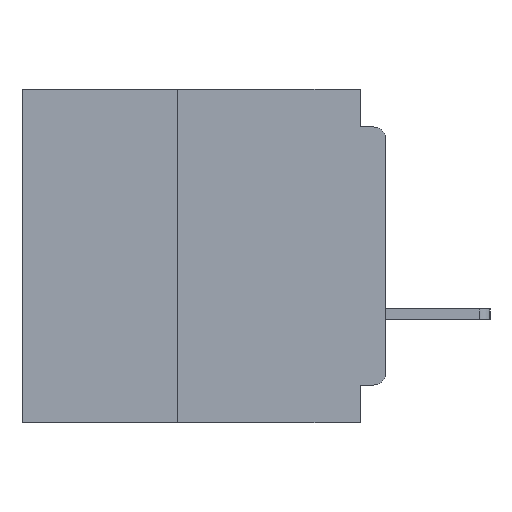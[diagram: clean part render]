
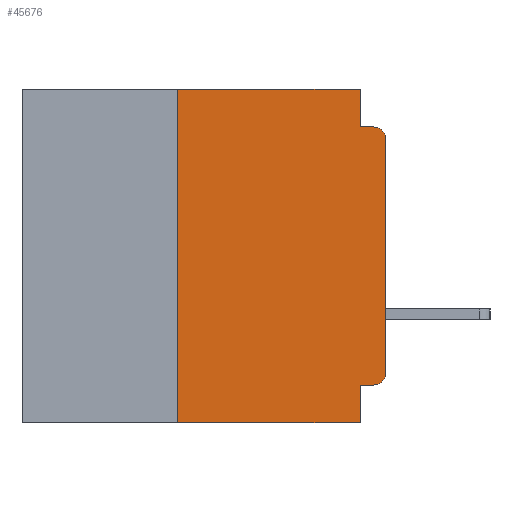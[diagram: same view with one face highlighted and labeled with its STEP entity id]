
A CAD part, left-side view. The second image highlights one B-rep face of the part: STEP entity #45676.
In plain terms, the highlighted planar face has unit normal (-1, 0, 0).
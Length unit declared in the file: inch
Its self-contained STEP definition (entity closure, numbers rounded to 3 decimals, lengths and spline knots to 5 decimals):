
#1343 = VECTOR ( 'NONE', #16385, 39.37008 ) ;
#1486 = CARTESIAN_POINT ( 'NONE',  ( 0., 0., -0.34 ) ) ;
#1702 = CARTESIAN_POINT ( 'NONE',  ( 0., 0.437, -0.4 ) ) ;
#2085 = CARTESIAN_POINT ( 'NONE',  ( 0., 0., -0.06 ) ) ;
#2551 = ORIENTED_EDGE ( 'NONE', *, *, #31045, .T. ) ;
#2575 = VERTEX_POINT ( 'NONE', #42273 ) ;
#2847 = CIRCLE ( 'NONE', #25628, 0.015 ) ;
#3550 = VERTEX_POINT ( 'NONE', #44899 ) ;
#4883 = ORIENTED_EDGE ( 'NONE', *, *, #26939, .T. ) ;
#7940 = CARTESIAN_POINT ( 'NONE',  ( 0., 0.25, -0.4 ) ) ;
#8504 = CARTESIAN_POINT ( 'NONE',  ( 0., 0.437, 0. ) ) ;
#9135 = CARTESIAN_POINT ( 'NONE',  ( 0., 0., -0.045 ) ) ;
#9590 = FACE_OUTER_BOUND ( 'NONE', #31355, .T. ) ;
#10597 = CARTESIAN_POINT ( 'NONE',  ( 0., 0.015, -0.34 ) ) ;
#11139 = CARTESIAN_POINT ( 'NONE',  ( 0., 0.015, -0.355 ) ) ;
#11684 = DIRECTION ( 'NONE',  ( 0., 0., -1. ) ) ;
#11767 = DIRECTION ( 'NONE',  ( 0., 0., 1. ) ) ;
#12786 = VERTEX_POINT ( 'NONE', #33466 ) ;
#12828 = DIRECTION ( 'NONE',  ( 0., -1., 0. ) ) ;
#13458 = DIRECTION ( 'NONE',  ( 0., -1., 0. ) ) ;
#14938 = DIRECTION ( 'NONE',  ( 0., 0., -1. ) ) ;
#15249 = EDGE_CURVE ( 'NONE', #35882, #40280, #45201, .T. ) ;
#16385 = DIRECTION ( 'NONE',  ( 0., 0., 1. ) ) ;
#16493 = AXIS2_PLACEMENT_3D ( 'NONE', #20084, #37190, #11684 ) ;
#18243 = VECTOR ( 'NONE', #52682, 39.37008 ) ;
#19333 = CARTESIAN_POINT ( 'NONE',  ( 0., 0.015, -0.06 ) ) ;
#20084 = CARTESIAN_POINT ( 'NONE',  ( 0., 0.437, 0. ) ) ;
#20311 = VERTEX_POINT ( 'NONE', #2085 ) ;
#21010 = DIRECTION ( 'NONE',  ( 0., 1., 0. ) ) ;
#22916 = DIRECTION ( 'NONE',  ( 0., -1., 0. ) ) ;
#23565 = DIRECTION ( 'NONE',  ( 0., 0., -1. ) ) ;
#23844 = VERTEX_POINT ( 'NONE', #30542 ) ;
#25628 = AXIS2_PLACEMENT_3D ( 'NONE', #10597, #40368, #14938 ) ;
#26117 = VECTOR ( 'NONE', #13458, 39.37008 ) ;
#26939 = EDGE_CURVE ( 'NONE', #43745, #46457, #2847, .T. ) ;
#28578 = ORIENTED_EDGE ( 'NONE', *, *, #34193, .T. ) ;
#30542 = CARTESIAN_POINT ( 'NONE',  ( 0., 0.031, 0. ) ) ;
#31045 = EDGE_CURVE ( 'NONE', #46457, #20311, #47578, .T. ) ;
#31355 = EDGE_LOOP ( 'NONE', ( #2551, #28578, #42741, #45619, #48476, #47615, #47704, #32924, #36792, #4883 ) ) ;
#31519 = CARTESIAN_POINT ( 'NONE',  ( 0., 0.031, -0.045 ) ) ;
#32924 = ORIENTED_EDGE ( 'NONE', *, *, #46124, .F. ) ;
#33305 = EDGE_CURVE ( 'NONE', #37287, #3550, #40085, .T. ) ;
#33466 = CARTESIAN_POINT ( 'NONE',  ( 0., 0.031, -0.355 ) ) ;
#33899 = LINE ( 'NONE', #42177, #35237 ) ;
#34193 = EDGE_CURVE ( 'NONE', #20311, #3550, #47916, .T. ) ;
#35237 = VECTOR ( 'NONE', #21010, 39.37008 ) ;
#35882 = VERTEX_POINT ( 'NONE', #51543 ) ;
#36351 = CARTESIAN_POINT ( 'NONE',  ( 0., 0.031, 0. ) ) ;
#36402 = VECTOR ( 'NONE', #11767, 39.37008 ) ;
#36792 = ORIENTED_EDGE ( 'NONE', *, *, #41934, .F. ) ;
#36910 = VECTOR ( 'NONE', #53026, 39.37008 ) ;
#37190 = DIRECTION ( 'NONE',  ( 1., 0., 0. ) ) ;
#37287 = VERTEX_POINT ( 'NONE', #31519 ) ;
#39342 = EDGE_CURVE ( 'NONE', #23844, #37287, #49363, .T. ) ;
#40085 = LINE ( 'NONE', #9135, #26117 ) ;
#40280 = VERTEX_POINT ( 'NONE', #42901 ) ;
#40368 = DIRECTION ( 'NONE',  ( -1., 0., 0. ) ) ;
#41226 = VECTOR ( 'NONE', #12828, 39.37008 ) ;
#41525 = CARTESIAN_POINT ( 'NONE',  ( 0., 0., 0. ) ) ;
#41934 = EDGE_CURVE ( 'NONE', #43745, #12786, #33899, .T. ) ;
#41965 = EDGE_CURVE ( 'NONE', #40280, #23844, #42528, .T. ) ;
#42177 = CARTESIAN_POINT ( 'NONE',  ( 0., 0., -0.355 ) ) ;
#42273 = CARTESIAN_POINT ( 'NONE',  ( 0., 0.031, -0.4 ) ) ;
#42528 = LINE ( 'NONE', #8504, #41226 ) ;
#42741 = ORIENTED_EDGE ( 'NONE', *, *, #33305, .F. ) ;
#42901 = CARTESIAN_POINT ( 'NONE',  ( 0., 0.25, 0. ) ) ;
#43745 = VERTEX_POINT ( 'NONE', #11139 ) ;
#44899 = CARTESIAN_POINT ( 'NONE',  ( 0., 0.015, -0.045 ) ) ;
#45201 = LINE ( 'NONE', #7940, #1343 ) ;
#45619 = ORIENTED_EDGE ( 'NONE', *, *, #39342, .F. ) ;
#45676 = ADVANCED_FACE ( 'NONE', ( #9590 ), #49621, .F. ) ;
#46124 = EDGE_CURVE ( 'NONE', #12786, #2575, #51906, .T. ) ;
#46457 = VERTEX_POINT ( 'NONE', #1486 ) ;
#47578 = LINE ( 'NONE', #41525, #36402 ) ;
#47615 = ORIENTED_EDGE ( 'NONE', *, *, #15249, .F. ) ;
#47704 = ORIENTED_EDGE ( 'NONE', *, *, #53986, .T. ) ;
#47916 = CIRCLE ( 'NONE', #48204, 0.015 ) ;
#48204 = AXIS2_PLACEMENT_3D ( 'NONE', #19333, #48881, #23565 ) ;
#48476 = ORIENTED_EDGE ( 'NONE', *, *, #41965, .F. ) ;
#48487 = CARTESIAN_POINT ( 'NONE',  ( 0., 0.031, -0.4 ) ) ;
#48881 = DIRECTION ( 'NONE',  ( -1., 0., 0. ) ) ;
#49363 = LINE ( 'NONE', #36351, #36910 ) ;
#49621 = PLANE ( 'NONE',  #16493 ) ;
#50468 = LINE ( 'NONE', #1702, #51774 ) ;
#51543 = CARTESIAN_POINT ( 'NONE',  ( 0., 0.25, -0.4 ) ) ;
#51774 = VECTOR ( 'NONE', #22916, 39.37008 ) ;
#51906 = LINE ( 'NONE', #48487, #18243 ) ;
#52682 = DIRECTION ( 'NONE',  ( 0., 0., -1. ) ) ;
#53026 = DIRECTION ( 'NONE',  ( 0., 0., -1. ) ) ;
#53986 = EDGE_CURVE ( 'NONE', #35882, #2575, #50468, .T. ) ;
